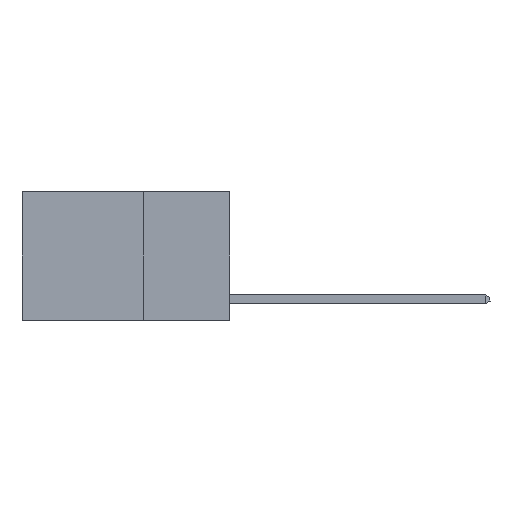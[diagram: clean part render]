
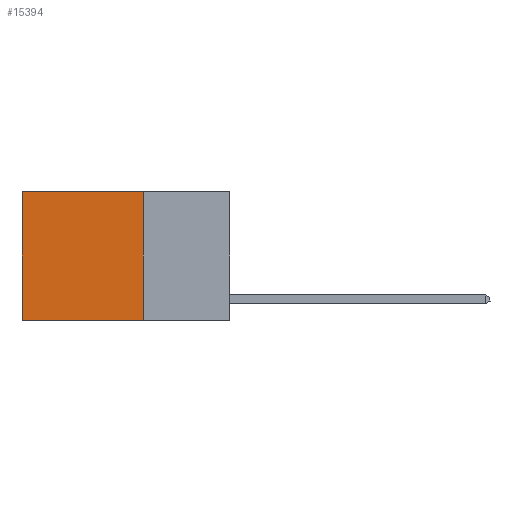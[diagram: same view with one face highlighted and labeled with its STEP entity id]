
A CAD part, left-side view. The second image highlights one B-rep face of the part: STEP entity #15394.
In plain terms, the highlighted planar face has unit normal (-1, 0, 0).
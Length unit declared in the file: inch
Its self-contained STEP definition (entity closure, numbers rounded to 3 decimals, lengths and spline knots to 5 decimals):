
#1253 = CARTESIAN_POINT ( 'NONE',  ( 0.2625, 0.6, -0.37 ) ) ;
#1442 = LINE ( 'NONE', #16853, #11837 ) ;
#1788 = ORIENTED_EDGE ( 'NONE', *, *, #12766, .F. ) ;
#2164 = DIRECTION ( 'NONE',  ( 1., 0., 0. ) ) ;
#3246 = VECTOR ( 'NONE', #16705, 39.37008 ) ;
#5303 = ORIENTED_EDGE ( 'NONE', *, *, #10569, .T. ) ;
#5840 = ORIENTED_EDGE ( 'NONE', *, *, #8370, .T. ) ;
#5946 = VERTEX_POINT ( 'NONE', #7205 ) ;
#6516 = VECTOR ( 'NONE', #9044, 39.37008 ) ;
#7160 = CARTESIAN_POINT ( 'NONE',  ( 0.2625, 0.6, 0. ) ) ;
#7205 = CARTESIAN_POINT ( 'NONE',  ( 0.2625, 0.6, 0. ) ) ;
#7884 = ORIENTED_EDGE ( 'NONE', *, *, #10906, .F. ) ;
#8370 = EDGE_CURVE ( 'NONE', #5946, #15609, #10423, .T. ) ;
#8874 = PLANE ( 'NONE',  #15272 ) ;
#9044 = DIRECTION ( 'NONE',  ( 0., 1., 0. ) ) ;
#9118 = CARTESIAN_POINT ( 'NONE',  ( 0.2625, 0.25, 0. ) ) ;
#9277 = LINE ( 'NONE', #17131, #6516 ) ;
#9468 = EDGE_LOOP ( 'NONE', ( #5840, #1788, #7884, #5303 ) ) ;
#10233 = CARTESIAN_POINT ( 'NONE',  ( 0.2625, 0.25, 0. ) ) ;
#10395 = CARTESIAN_POINT ( 'NONE',  ( 0.2625, 0.25, -0.37 ) ) ;
#10423 = LINE ( 'NONE', #7160, #3246 ) ;
#10557 = LINE ( 'NONE', #9118, #13791 ) ;
#10569 = EDGE_CURVE ( 'NONE', #13868, #5946, #10557, .T. ) ;
#10906 = EDGE_CURVE ( 'NONE', #13868, #11704, #1442, .T. ) ;
#11619 = DIRECTION ( 'NONE',  ( 0., 0., -1. ) ) ;
#11704 = VERTEX_POINT ( 'NONE', #10395 ) ;
#11728 = FACE_OUTER_BOUND ( 'NONE', #9468, .T. ) ;
#11837 = VECTOR ( 'NONE', #14194, 39.37008 ) ;
#12766 = EDGE_CURVE ( 'NONE', #11704, #15609, #9277, .T. ) ;
#13791 = VECTOR ( 'NONE', #15884, 39.37008 ) ;
#13868 = VERTEX_POINT ( 'NONE', #15117 ) ;
#14194 = DIRECTION ( 'NONE',  ( 0., 0., -1. ) ) ;
#15117 = CARTESIAN_POINT ( 'NONE',  ( 0.2625, 0.25, 0. ) ) ;
#15272 = AXIS2_PLACEMENT_3D ( 'NONE', #10233, #2164, #11619 ) ;
#15394 = ADVANCED_FACE ( 'NONE', ( #11728 ), #8874, .F. ) ;
#15609 = VERTEX_POINT ( 'NONE', #1253 ) ;
#15884 = DIRECTION ( 'NONE',  ( 0., 1., 0. ) ) ;
#16705 = DIRECTION ( 'NONE',  ( 0., 0., -1. ) ) ;
#16853 = CARTESIAN_POINT ( 'NONE',  ( 0.2625, 0.25, 0. ) ) ;
#17131 = CARTESIAN_POINT ( 'NONE',  ( 0.2625, 0.25, -0.37 ) ) ;
